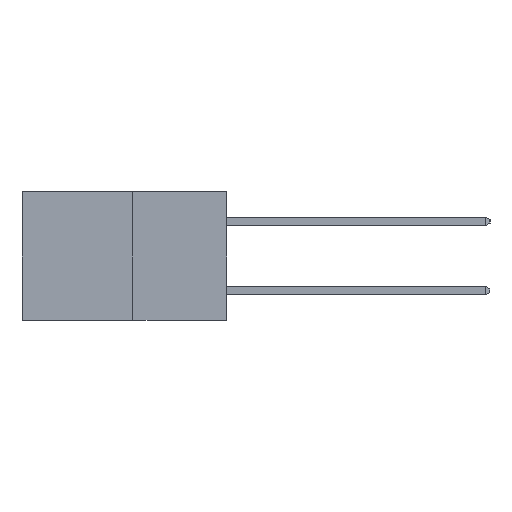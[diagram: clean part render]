
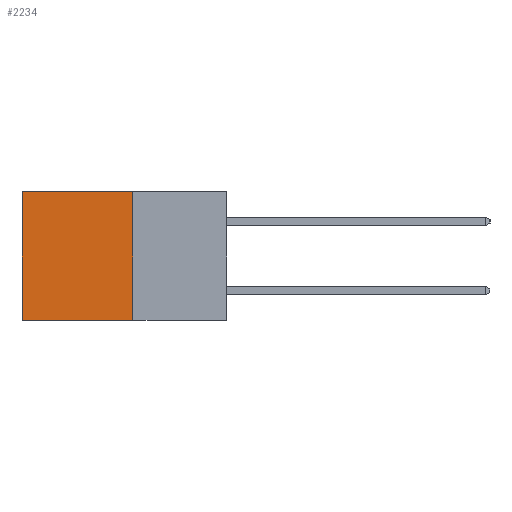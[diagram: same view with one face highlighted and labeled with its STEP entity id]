
A CAD part, left-side view. The second image highlights one B-rep face of the part: STEP entity #2234.
In plain terms, the highlighted planar face has unit normal (-1, 0, 0).
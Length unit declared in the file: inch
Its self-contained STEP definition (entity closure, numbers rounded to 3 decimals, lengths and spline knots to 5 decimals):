
#185 = EDGE_CURVE ( 'NONE', #6816, #9078, #18252, .T. ) ;
#1326 = ORIENTED_EDGE ( 'NONE', *, *, #16906, .T. ) ;
#2234 = ADVANCED_FACE ( 'NONE', ( #19856 ), #22688, .F. ) ;
#2462 = ORIENTED_EDGE ( 'NONE', *, *, #3869, .T. ) ;
#2517 = ORIENTED_EDGE ( 'NONE', *, *, #185, .F. ) ;
#2595 = DIRECTION ( 'NONE',  ( 0., 1., 0. ) ) ;
#3377 = ORIENTED_EDGE ( 'NONE', *, *, #13890, .F. ) ;
#3743 = CARTESIAN_POINT ( 'NONE',  ( 0.277, 0.27, 0. ) ) ;
#3869 = EDGE_CURVE ( 'NONE', #14152, #20210, #15380, .T. ) ;
#4488 = DIRECTION ( 'NONE',  ( 0., 0., -1. ) ) ;
#5701 = CARTESIAN_POINT ( 'NONE',  ( 0.277, 0.59, 0. ) ) ;
#6816 = VERTEX_POINT ( 'NONE', #3743 ) ;
#8267 = CARTESIAN_POINT ( 'NONE',  ( 0.277, 0.27, -0.37 ) ) ;
#9078 = VERTEX_POINT ( 'NONE', #10155 ) ;
#9898 = DIRECTION ( 'NONE',  ( 0., 1., 0. ) ) ;
#10155 = CARTESIAN_POINT ( 'NONE',  ( 0.277, 0.27, -0.37 ) ) ;
#11345 = DIRECTION ( 'NONE',  ( 1., 0., 0. ) ) ;
#12134 = VECTOR ( 'NONE', #2595, 39.37008 ) ;
#12788 = CARTESIAN_POINT ( 'NONE',  ( 0.277, 0.59, -0.37 ) ) ;
#13890 = EDGE_CURVE ( 'NONE', #9078, #20210, #17004, .T. ) ;
#14152 = VERTEX_POINT ( 'NONE', #5701 ) ;
#14811 = VECTOR ( 'NONE', #4488, 39.37008 ) ;
#15380 = LINE ( 'NONE', #12788, #14811 ) ;
#16322 = VECTOR ( 'NONE', #9898, 39.37008 ) ;
#16875 = LINE ( 'NONE', #20801, #16322 ) ;
#16906 = EDGE_CURVE ( 'NONE', #6816, #14152, #16875, .T. ) ;
#17004 = LINE ( 'NONE', #8267, #12134 ) ;
#17339 = AXIS2_PLACEMENT_3D ( 'NONE', #22244, #11345, #22240 ) ;
#18252 = LINE ( 'NONE', #19114, #18808 ) ;
#18808 = VECTOR ( 'NONE', #19168, 39.37008 ) ;
#19114 = CARTESIAN_POINT ( 'NONE',  ( 0.277, 0.27, -0.37 ) ) ;
#19168 = DIRECTION ( 'NONE',  ( 0., 0., -1. ) ) ;
#19856 = FACE_OUTER_BOUND ( 'NONE', #22994, .T. ) ;
#20210 = VERTEX_POINT ( 'NONE', #22124 ) ;
#20801 = CARTESIAN_POINT ( 'NONE',  ( 0.277, 0.27, 0. ) ) ;
#22124 = CARTESIAN_POINT ( 'NONE',  ( 0.277, 0.59, -0.37 ) ) ;
#22240 = DIRECTION ( 'NONE',  ( 0., 0., -1. ) ) ;
#22244 = CARTESIAN_POINT ( 'NONE',  ( 0.277, 0.27, -0.37 ) ) ;
#22688 = PLANE ( 'NONE',  #17339 ) ;
#22994 = EDGE_LOOP ( 'NONE', ( #2462, #3377, #2517, #1326 ) ) ;
